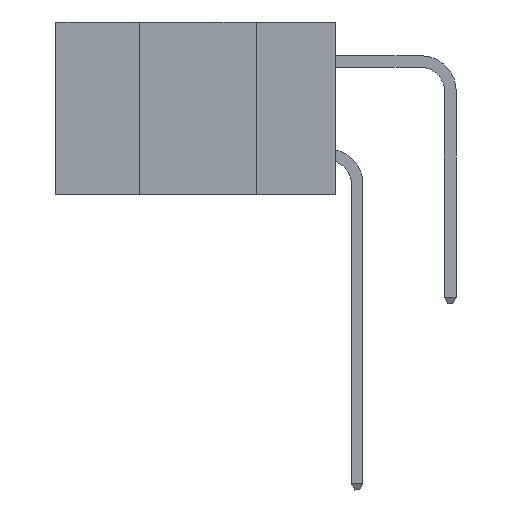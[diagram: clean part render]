
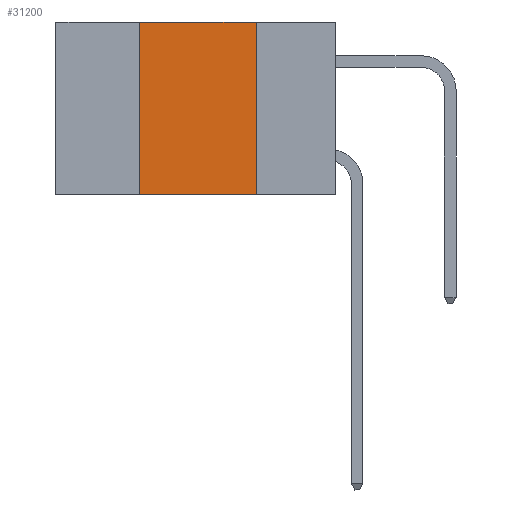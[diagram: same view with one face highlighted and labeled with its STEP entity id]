
A CAD part, left-side view. The second image highlights one B-rep face of the part: STEP entity #31200.
In plain terms, the highlighted planar face has unit normal (-1, 0, 0).
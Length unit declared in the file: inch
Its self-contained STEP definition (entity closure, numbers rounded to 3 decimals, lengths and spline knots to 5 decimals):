
#12 = VECTOR ( 'NONE', #2019, 39.37008 ) ;
#667 = CARTESIAN_POINT ( 'NONE',  ( 0., 0.42, 0. ) ) ;
#780 = ORIENTED_EDGE ( 'NONE', *, *, #28592, .F. ) ;
#1767 = LINE ( 'NONE', #24602, #25175 ) ;
#2019 = DIRECTION ( 'NONE',  ( 0., 0., -1. ) ) ;
#3329 = VERTEX_POINT ( 'NONE', #24533 ) ;
#3997 = VECTOR ( 'NONE', #5498, 39.37008 ) ;
#4282 = CARTESIAN_POINT ( 'NONE',  ( 0., 0.6, 0. ) ) ;
#4501 = ORIENTED_EDGE ( 'NONE', *, *, #20253, .F. ) ;
#4799 = ORIENTED_EDGE ( 'NONE', *, *, #23351, .T. ) ;
#4935 = ORIENTED_EDGE ( 'NONE', *, *, #30862, .F. ) ;
#5090 = CARTESIAN_POINT ( 'NONE',  ( 0., 0.17, -0.37 ) ) ;
#5498 = DIRECTION ( 'NONE',  ( 0., -1., 0. ) ) ;
#5983 = FACE_OUTER_BOUND ( 'NONE', #30211, .T. ) ;
#10215 = DIRECTION ( 'NONE',  ( 1., 0., 0. ) ) ;
#11957 = VERTEX_POINT ( 'NONE', #21276 ) ;
#12061 = LINE ( 'NONE', #25363, #12 ) ;
#12298 = PLANE ( 'NONE',  #35393 ) ;
#13817 = LINE ( 'NONE', #667, #33861 ) ;
#20253 = EDGE_CURVE ( 'NONE', #11957, #3329, #1767, .T. ) ;
#21276 = CARTESIAN_POINT ( 'NONE',  ( 0., 0.42, 0. ) ) ;
#22008 = DIRECTION ( 'NONE',  ( 0., 0., -1. ) ) ;
#22341 = VERTEX_POINT ( 'NONE', #5090 ) ;
#23062 = CARTESIAN_POINT ( 'NONE',  ( 0., 0.6, -0.37 ) ) ;
#23351 = EDGE_CURVE ( 'NONE', #32732, #22341, #23737, .T. ) ;
#23737 = LINE ( 'NONE', #23062, #3997 ) ;
#24533 = CARTESIAN_POINT ( 'NONE',  ( 0., 0.17, 0. ) ) ;
#24602 = CARTESIAN_POINT ( 'NONE',  ( 0., 0.6, 0. ) ) ;
#25175 = VECTOR ( 'NONE', #36468, 39.37008 ) ;
#25363 = CARTESIAN_POINT ( 'NONE',  ( 0., 0.17, 0. ) ) ;
#28592 = EDGE_CURVE ( 'NONE', #32732, #11957, #13817, .T. ) ;
#30211 = EDGE_LOOP ( 'NONE', ( #4935, #4501, #780, #4799 ) ) ;
#30862 = EDGE_CURVE ( 'NONE', #3329, #22341, #12061, .T. ) ;
#31200 = ADVANCED_FACE ( 'NONE', ( #5983 ), #12298, .F. ) ;
#32732 = VERTEX_POINT ( 'NONE', #35726 ) ;
#33861 = VECTOR ( 'NONE', #36016, 39.37008 ) ;
#35393 = AXIS2_PLACEMENT_3D ( 'NONE', #4282, #10215, #22008 ) ;
#35726 = CARTESIAN_POINT ( 'NONE',  ( 0., 0.42, -0.37 ) ) ;
#36016 = DIRECTION ( 'NONE',  ( 0., 0., 1. ) ) ;
#36468 = DIRECTION ( 'NONE',  ( 0., -1., 0. ) ) ;
